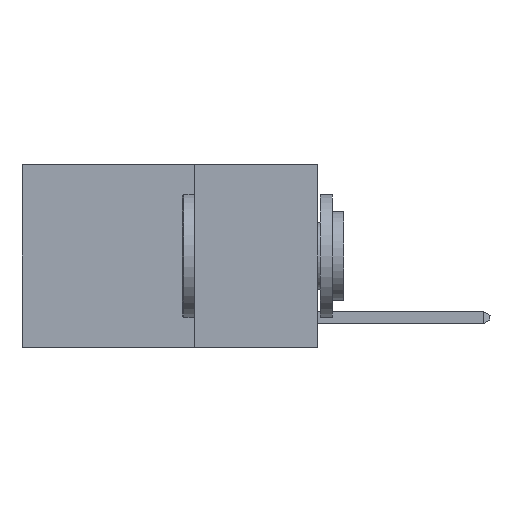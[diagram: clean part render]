
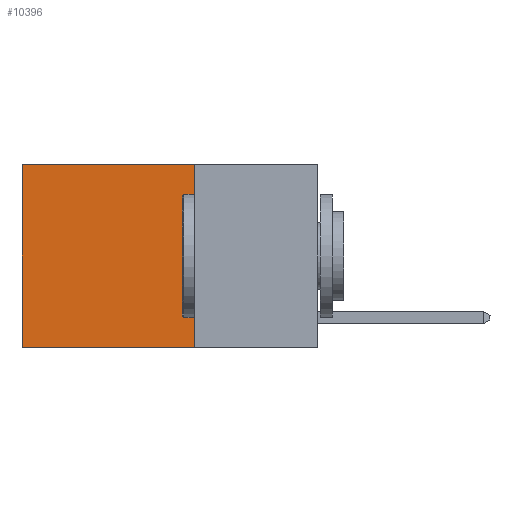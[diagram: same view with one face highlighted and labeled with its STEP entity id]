
A CAD part, left-side view. The second image highlights one B-rep face of the part: STEP entity #10396.
In plain terms, the highlighted planar face has unit normal (-1, 0, 0).
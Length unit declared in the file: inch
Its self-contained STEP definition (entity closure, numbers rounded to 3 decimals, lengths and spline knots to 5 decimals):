
#824 = FACE_OUTER_BOUND ( 'NONE', #2918, .T. ) ;
#834 = VECTOR ( 'NONE', #10514, 39.37008 ) ;
#841 = CARTESIAN_POINT ( 'NONE',  ( 0.2625, 0.25, 0. ) ) ;
#1684 = VERTEX_POINT ( 'NONE', #22565 ) ;
#1766 = CARTESIAN_POINT ( 'NONE',  ( 0.2625, 0.25, -0.37 ) ) ;
#2166 = LINE ( 'NONE', #8057, #4544 ) ;
#2293 = CARTESIAN_POINT ( 'NONE',  ( 0.2625, 0.25, 0. ) ) ;
#2741 = ORIENTED_EDGE ( 'NONE', *, *, #4916, .F. ) ;
#2833 = CARTESIAN_POINT ( 'NONE',  ( 0.2625, 0.25, -0.37 ) ) ;
#2918 = EDGE_LOOP ( 'NONE', ( #21406, #2741, #14208, #17514 ) ) ;
#3396 = VECTOR ( 'NONE', #6253, 39.37008 ) ;
#3761 = CARTESIAN_POINT ( 'NONE',  ( 0.2625, 0.6, -0.37 ) ) ;
#4544 = VECTOR ( 'NONE', #6009, 39.37008 ) ;
#4916 = EDGE_CURVE ( 'NONE', #10600, #6671, #8497, .T. ) ;
#5648 = CARTESIAN_POINT ( 'NONE',  ( 0.2625, 0.25, 0. ) ) ;
#5711 = AXIS2_PLACEMENT_3D ( 'NONE', #2293, #8176, #15480 ) ;
#6009 = DIRECTION ( 'NONE',  ( 0., 0., -1. ) ) ;
#6253 = DIRECTION ( 'NONE',  ( 0., 0., -1. ) ) ;
#6671 = VERTEX_POINT ( 'NONE', #3761 ) ;
#8057 = CARTESIAN_POINT ( 'NONE',  ( 0.2625, 0.25, 0. ) ) ;
#8176 = DIRECTION ( 'NONE',  ( 1., 0., 0. ) ) ;
#8497 = LINE ( 'NONE', #2833, #834 ) ;
#8930 = EDGE_CURVE ( 'NONE', #15495, #10600, #2166, .T. ) ;
#9136 = DIRECTION ( 'NONE',  ( 0., 1., 0. ) ) ;
#9973 = CARTESIAN_POINT ( 'NONE',  ( 0.2625, 0.6, 0. ) ) ;
#10396 = ADVANCED_FACE ( 'NONE', ( #824 ), #11410, .F. ) ;
#10514 = DIRECTION ( 'NONE',  ( 0., 1., 0. ) ) ;
#10600 = VERTEX_POINT ( 'NONE', #1766 ) ;
#11410 = PLANE ( 'NONE',  #5711 ) ;
#12005 = LINE ( 'NONE', #9973, #3396 ) ;
#14208 = ORIENTED_EDGE ( 'NONE', *, *, #8930, .F. ) ;
#15480 = DIRECTION ( 'NONE',  ( 0., 0., -1. ) ) ;
#15495 = VERTEX_POINT ( 'NONE', #841 ) ;
#16938 = LINE ( 'NONE', #5648, #21073 ) ;
#17514 = ORIENTED_EDGE ( 'NONE', *, *, #21365, .T. ) ;
#19416 = EDGE_CURVE ( 'NONE', #1684, #6671, #12005, .T. ) ;
#21073 = VECTOR ( 'NONE', #9136, 39.37008 ) ;
#21365 = EDGE_CURVE ( 'NONE', #15495, #1684, #16938, .T. ) ;
#21406 = ORIENTED_EDGE ( 'NONE', *, *, #19416, .T. ) ;
#22565 = CARTESIAN_POINT ( 'NONE',  ( 0.2625, 0.6, 0. ) ) ;
